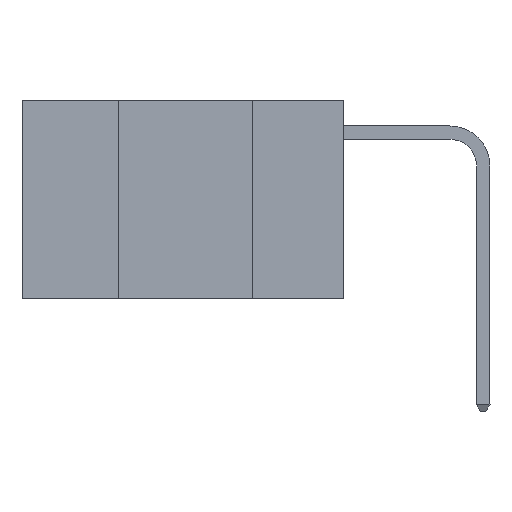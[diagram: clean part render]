
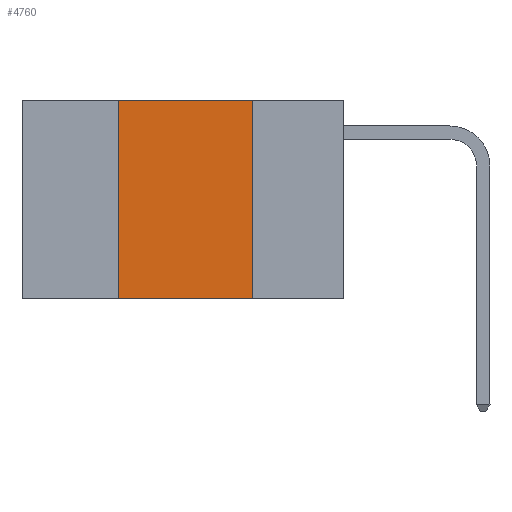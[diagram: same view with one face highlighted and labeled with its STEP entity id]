
A CAD part, left-side view. The second image highlights one B-rep face of the part: STEP entity #4760.
In plain terms, the highlighted planar face has unit normal (-1, 0, 0).
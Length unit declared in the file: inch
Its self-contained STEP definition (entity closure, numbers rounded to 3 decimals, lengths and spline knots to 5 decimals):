
#56 = VERTEX_POINT ( 'NONE', #11061 ) ;
#528 = LINE ( 'NONE', #11526, #16125 ) ;
#1466 = DIRECTION ( 'NONE',  ( 0., 0., -1. ) ) ;
#1655 = PLANE ( 'NONE',  #12744 ) ;
#2013 = DIRECTION ( 'NONE',  ( 0., 0., 1. ) ) ;
#2129 = ORIENTED_EDGE ( 'NONE', *, *, #18431, .T. ) ;
#2368 = FACE_OUTER_BOUND ( 'NONE', #16992, .T. ) ;
#2755 = ORIENTED_EDGE ( 'NONE', *, *, #14262, .F. ) ;
#3068 = EDGE_CURVE ( 'NONE', #9462, #4559, #528, .T. ) ;
#3084 = DIRECTION ( 'NONE',  ( 0., 0., -1. ) ) ;
#4559 = VERTEX_POINT ( 'NONE', #8116 ) ;
#4760 = ADVANCED_FACE ( 'NONE', ( #2368 ), #1655, .F. ) ;
#5394 = CARTESIAN_POINT ( 'NONE',  ( 0., 0.6, 0. ) ) ;
#5963 = LINE ( 'NONE', #5394, #13091 ) ;
#6822 = EDGE_CURVE ( 'NONE', #15221, #56, #8353, .T. ) ;
#7014 = DIRECTION ( 'NONE',  ( 0., -1., 0. ) ) ;
#7365 = CARTESIAN_POINT ( 'NONE',  ( 0., 0.6, 0. ) ) ;
#8116 = CARTESIAN_POINT ( 'NONE',  ( 0., 0.17, -0.37 ) ) ;
#8353 = LINE ( 'NONE', #14867, #15448 ) ;
#8569 = CARTESIAN_POINT ( 'NONE',  ( 0., 0.17, 0. ) ) ;
#9462 = VERTEX_POINT ( 'NONE', #8569 ) ;
#10638 = CARTESIAN_POINT ( 'NONE',  ( 0., 0.42, -0.37 ) ) ;
#10667 = ORIENTED_EDGE ( 'NONE', *, *, #6822, .F. ) ;
#11061 = CARTESIAN_POINT ( 'NONE',  ( 0., 0.42, 0. ) ) ;
#11526 = CARTESIAN_POINT ( 'NONE',  ( 0., 0.17, 0. ) ) ;
#11701 = DIRECTION ( 'NONE',  ( 1., 0., 0. ) ) ;
#12182 = ORIENTED_EDGE ( 'NONE', *, *, #3068, .F. ) ;
#12516 = VECTOR ( 'NONE', #7014, 39.37008 ) ;
#12744 = AXIS2_PLACEMENT_3D ( 'NONE', #7365, #11701, #3084 ) ;
#12950 = LINE ( 'NONE', #14086, #12516 ) ;
#13091 = VECTOR ( 'NONE', #16724, 39.37008 ) ;
#14086 = CARTESIAN_POINT ( 'NONE',  ( 0., 0.6, -0.37 ) ) ;
#14262 = EDGE_CURVE ( 'NONE', #56, #9462, #5963, .T. ) ;
#14867 = CARTESIAN_POINT ( 'NONE',  ( 0., 0.42, 0. ) ) ;
#15221 = VERTEX_POINT ( 'NONE', #10638 ) ;
#15448 = VECTOR ( 'NONE', #2013, 39.37008 ) ;
#16125 = VECTOR ( 'NONE', #1466, 39.37008 ) ;
#16724 = DIRECTION ( 'NONE',  ( 0., -1., 0. ) ) ;
#16992 = EDGE_LOOP ( 'NONE', ( #12182, #2755, #10667, #2129 ) ) ;
#18431 = EDGE_CURVE ( 'NONE', #15221, #4559, #12950, .T. ) ;
